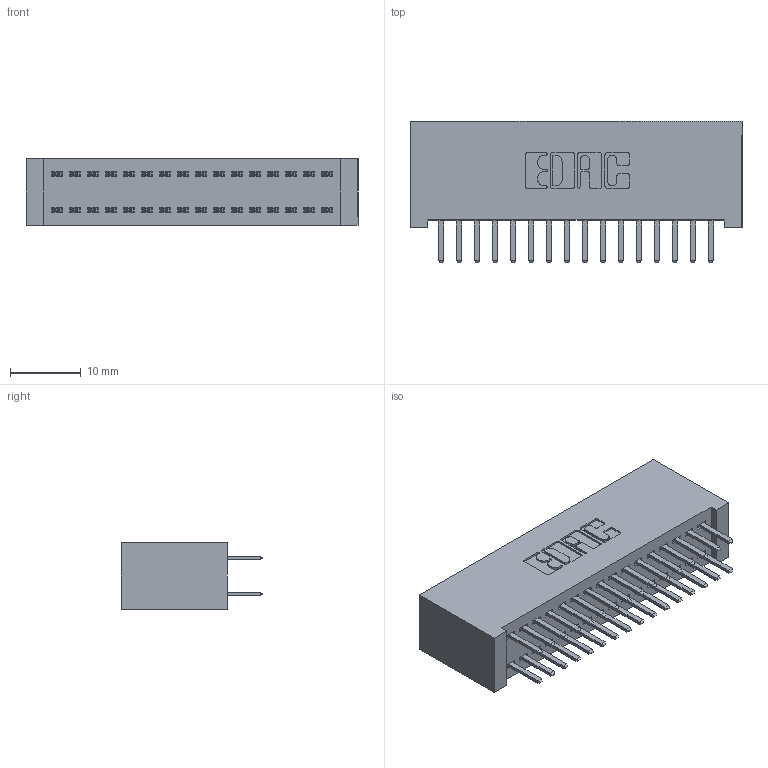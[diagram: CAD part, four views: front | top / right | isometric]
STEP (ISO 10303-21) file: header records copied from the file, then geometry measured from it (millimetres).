
FILE_DESCRIPTION (( 'STEP AP203' ), '1' );
FILE_NAME ('392-032-520-201.STEP', '2018-08-15T23:34:09', ( '' ), ( '' ), 'SwSTEP 2.0', 'SolidWorks 2016', '' );
FILE_SCHEMA (( 'CONFIG_CONTROL_DESIGN' ));
Length unit declared in the file: inch
Products named in the file (3): 342 Part_Lugless; 345-292-001_345-293-120; 392-032-520-201
Assembly tree (33 placements, depth 2):
  392-032-520-201
    342 Part_Lugless
    345-292-001_345-293-120  x32
Bounding box: 46.89 x 20.02 x 9.4 mm (x, y, z)
Volume: 4515.3 mm3; surface area: 7122.2 mm2
Topology: 33 solids, 33 shells, 1894 faces, 5491 edges, 3574 vertices
Faces by surface type: plane 1278, cylinder 616
Entity records: 13361 total; most frequent: CARTESIAN_POINT 2254, ORIENTED_EDGE 2178, DIRECTION 1953, EDGE_CURVE 1089, VECTOR 965, LINE 965, VERTEX_POINT 722, AXIS2_PLACEMENT_3D 494
